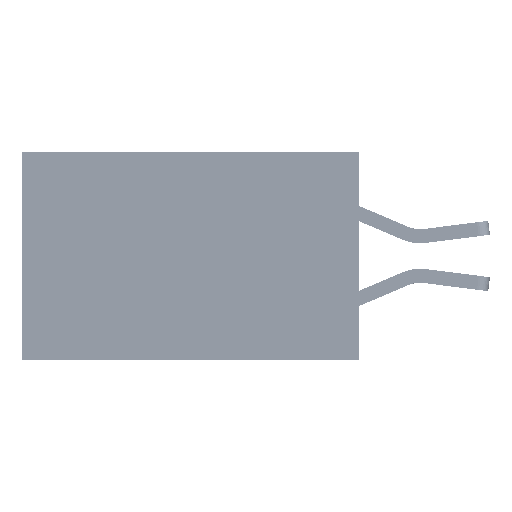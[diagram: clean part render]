
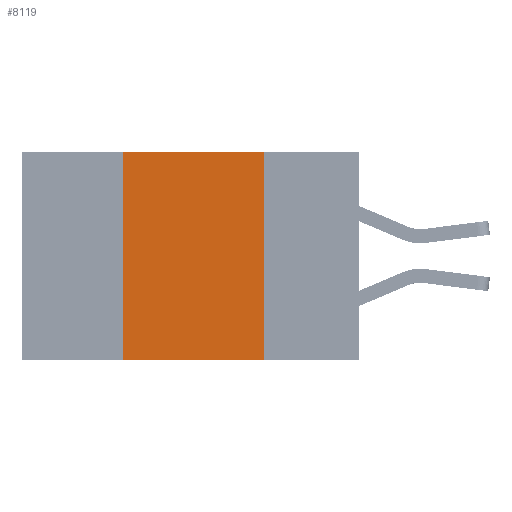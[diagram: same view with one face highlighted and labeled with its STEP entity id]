
A CAD part, left-side view. The second image highlights one B-rep face of the part: STEP entity #8119.
In plain terms, the highlighted planar face has unit normal (-1, 0, 0).
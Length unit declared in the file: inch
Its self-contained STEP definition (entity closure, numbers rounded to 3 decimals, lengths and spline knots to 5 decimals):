
#1457 = PLANE ( 'NONE',  #24599 ) ;
#3541 = ORIENTED_EDGE ( 'NONE', *, *, #20304, .F. ) ;
#4316 = VECTOR ( 'NONE', #21644, 39.37008 ) ;
#5378 = LINE ( 'NONE', #33572, #38272 ) ;
#5483 = CARTESIAN_POINT ( 'NONE',  ( 0., 0.17, -0.37 ) ) ;
#6467 = CARTESIAN_POINT ( 'NONE',  ( 0., 0.42, -0.37 ) ) ;
#8119 = ADVANCED_FACE ( 'NONE', ( #34077 ), #1457, .F. ) ;
#8151 = ORIENTED_EDGE ( 'NONE', *, *, #37487, .F. ) ;
#8277 = DIRECTION ( 'NONE',  ( 0., 0., -1. ) ) ;
#8957 = EDGE_LOOP ( 'NONE', ( #35232, #3541, #8151, #38657 ) ) ;
#10866 = EDGE_CURVE ( 'NONE', #22744, #15789, #25852, .T. ) ;
#15789 = VERTEX_POINT ( 'NONE', #5483 ) ;
#15889 = LINE ( 'NONE', #32637, #30603 ) ;
#18363 = VECTOR ( 'NONE', #40935, 39.37008 ) ;
#20304 = EDGE_CURVE ( 'NONE', #27047, #22744, #15889, .T. ) ;
#21644 = DIRECTION ( 'NONE',  ( 0., 0., -1. ) ) ;
#22744 = VERTEX_POINT ( 'NONE', #40506 ) ;
#23110 = CARTESIAN_POINT ( 'NONE',  ( 0., 0.6, -0.37 ) ) ;
#24599 = AXIS2_PLACEMENT_3D ( 'NONE', #41082, #26752, #8277 ) ;
#25852 = LINE ( 'NONE', #43600, #4316 ) ;
#26752 = DIRECTION ( 'NONE',  ( 1., 0., 0. ) ) ;
#27047 = VERTEX_POINT ( 'NONE', #44891 ) ;
#30064 = VERTEX_POINT ( 'NONE', #6467 ) ;
#30603 = VECTOR ( 'NONE', #36419, 39.37008 ) ;
#32637 = CARTESIAN_POINT ( 'NONE',  ( 0., 0.6, 0. ) ) ;
#33572 = CARTESIAN_POINT ( 'NONE',  ( 0., 0.42, 0. ) ) ;
#34077 = FACE_OUTER_BOUND ( 'NONE', #8957, .T. ) ;
#35232 = ORIENTED_EDGE ( 'NONE', *, *, #10866, .F. ) ;
#36419 = DIRECTION ( 'NONE',  ( 0., -1., 0. ) ) ;
#37487 = EDGE_CURVE ( 'NONE', #30064, #27047, #5378, .T. ) ;
#37524 = DIRECTION ( 'NONE',  ( 0., 0., 1. ) ) ;
#37985 = EDGE_CURVE ( 'NONE', #30064, #15789, #43945, .T. ) ;
#38272 = VECTOR ( 'NONE', #37524, 39.37008 ) ;
#38657 = ORIENTED_EDGE ( 'NONE', *, *, #37985, .T. ) ;
#40506 = CARTESIAN_POINT ( 'NONE',  ( 0., 0.17, 0. ) ) ;
#40935 = DIRECTION ( 'NONE',  ( 0., -1., 0. ) ) ;
#41082 = CARTESIAN_POINT ( 'NONE',  ( 0., 0.6, 0. ) ) ;
#43600 = CARTESIAN_POINT ( 'NONE',  ( 0., 0.17, 0. ) ) ;
#43945 = LINE ( 'NONE', #23110, #18363 ) ;
#44891 = CARTESIAN_POINT ( 'NONE',  ( 0., 0.42, 0. ) ) ;
